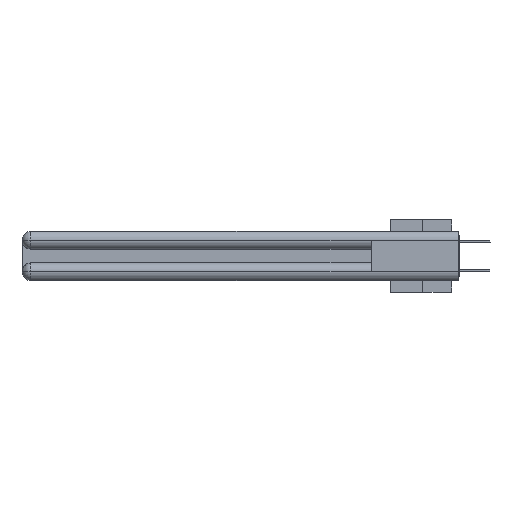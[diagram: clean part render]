
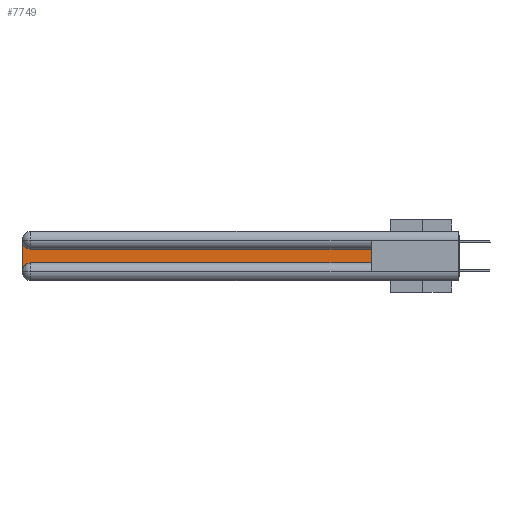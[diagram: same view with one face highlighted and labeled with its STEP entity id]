
A CAD part, left-side view. The second image highlights one B-rep face of the part: STEP entity #7749.
In plain terms, the highlighted planar face has unit normal (-1, 0, 0).
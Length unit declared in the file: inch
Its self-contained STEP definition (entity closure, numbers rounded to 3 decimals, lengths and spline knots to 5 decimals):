
#511 = CARTESIAN_POINT ( 'NONE',  ( 0.075, 3., -0.0625 ) ) ;
#866 = VECTOR ( 'NONE', #33618, 39.37008 ) ;
#921 = ORIENTED_EDGE ( 'NONE', *, *, #26251, .T. ) ;
#987 = CARTESIAN_POINT ( 'NONE',  ( 0.075, 2.94, -0.0625 ) ) ;
#1560 = AXIS2_PLACEMENT_3D ( 'NONE', #30135, #29956, #21166 ) ;
#2778 = CARTESIAN_POINT ( 'NONE',  ( 0.075, 2.94, -0.1225 ) ) ;
#4419 = CARTESIAN_POINT ( 'NONE',  ( 0.075, 0.6, -0.2175 ) ) ;
#4429 = LINE ( 'NONE', #22124, #866 ) ;
#5120 = LINE ( 'NONE', #17002, #17361 ) ;
#5468 = VECTOR ( 'NONE', #27698, 39.37008 ) ;
#7749 = ADVANCED_FACE ( 'NONE', ( #21948 ), #36551, .F. ) ;
#9212 = CARTESIAN_POINT ( 'NONE',  ( 0.075, 0.6, -0.2175 ) ) ;
#9612 = LINE ( 'NONE', #16049, #16347 ) ;
#10596 = VERTEX_POINT ( 'NONE', #24977 ) ;
#11991 = ORIENTED_EDGE ( 'NONE', *, *, #32189, .T. ) ;
#12304 = AXIS2_PLACEMENT_3D ( 'NONE', #27036, #23710, #33070 ) ;
#13868 = EDGE_LOOP ( 'NONE', ( #921, #34819, #21340, #28163, #23844, #11991 ) ) ;
#14079 = DIRECTION ( 'NONE',  ( 0., -1., 0. ) ) ;
#15265 = EDGE_CURVE ( 'NONE', #21096, #18859, #27298, .T. ) ;
#15394 = CIRCLE ( 'NONE', #12304, 0.06 ) ;
#16049 = CARTESIAN_POINT ( 'NONE',  ( 0.075, 3., -0.2175 ) ) ;
#16347 = VECTOR ( 'NONE', #27918, 39.37008 ) ;
#16528 = CARTESIAN_POINT ( 'NONE',  ( 0.075, 2.94, -0.2175 ) ) ;
#17002 = CARTESIAN_POINT ( 'NONE',  ( 0.075, 0.6, -0.2175 ) ) ;
#17361 = VECTOR ( 'NONE', #14079, 39.37008 ) ;
#18859 = VERTEX_POINT ( 'NONE', #511 ) ;
#21096 = VERTEX_POINT ( 'NONE', #2778 ) ;
#21166 = DIRECTION ( 'NONE',  ( 0., 0., -1. ) ) ;
#21340 = ORIENTED_EDGE ( 'NONE', *, *, #24192, .T. ) ;
#21461 = LINE ( 'NONE', #9212, #5468 ) ;
#21948 = FACE_OUTER_BOUND ( 'NONE', #13868, .T. ) ;
#22124 = CARTESIAN_POINT ( 'NONE',  ( 0.075, 0.6, -0.1225 ) ) ;
#23710 = DIRECTION ( 'NONE',  ( 1., 0., 0. ) ) ;
#23844 = ORIENTED_EDGE ( 'NONE', *, *, #38369, .T. ) ;
#24192 = EDGE_CURVE ( 'NONE', #18859, #10596, #9612, .T. ) ;
#24977 = CARTESIAN_POINT ( 'NONE',  ( 0.075, 3., -0.2775 ) ) ;
#25365 = VERTEX_POINT ( 'NONE', #16528 ) ;
#25754 = VERTEX_POINT ( 'NONE', #4419 ) ;
#26251 = EDGE_CURVE ( 'NONE', #35132, #21096, #4429, .T. ) ;
#27036 = CARTESIAN_POINT ( 'NONE',  ( 0.075, 2.94, -0.2775 ) ) ;
#27298 = CIRCLE ( 'NONE', #32271, 0.06 ) ;
#27698 = DIRECTION ( 'NONE',  ( 0., 0., 1. ) ) ;
#27918 = DIRECTION ( 'NONE',  ( 0., 0., -1. ) ) ;
#28163 = ORIENTED_EDGE ( 'NONE', *, *, #37100, .T. ) ;
#29956 = DIRECTION ( 'NONE',  ( 1., 0., 0. ) ) ;
#30135 = CARTESIAN_POINT ( 'NONE',  ( 0.075, 3., -0.1225 ) ) ;
#31131 = DIRECTION ( 'NONE',  ( 1., 0., 0. ) ) ;
#32149 = CARTESIAN_POINT ( 'NONE',  ( 0.075, 0.6, -0.1225 ) ) ;
#32189 = EDGE_CURVE ( 'NONE', #25754, #35132, #21461, .T. ) ;
#32271 = AXIS2_PLACEMENT_3D ( 'NONE', #987, #31131, #36783 ) ;
#33070 = DIRECTION ( 'NONE',  ( 0., 0., -1. ) ) ;
#33618 = DIRECTION ( 'NONE',  ( 0., 1., 0. ) ) ;
#34819 = ORIENTED_EDGE ( 'NONE', *, *, #15265, .T. ) ;
#35132 = VERTEX_POINT ( 'NONE', #32149 ) ;
#36551 = PLANE ( 'NONE',  #1560 ) ;
#36783 = DIRECTION ( 'NONE',  ( 0., 0., -1. ) ) ;
#37100 = EDGE_CURVE ( 'NONE', #10596, #25365, #15394, .T. ) ;
#38369 = EDGE_CURVE ( 'NONE', #25365, #25754, #5120, .T. ) ;
